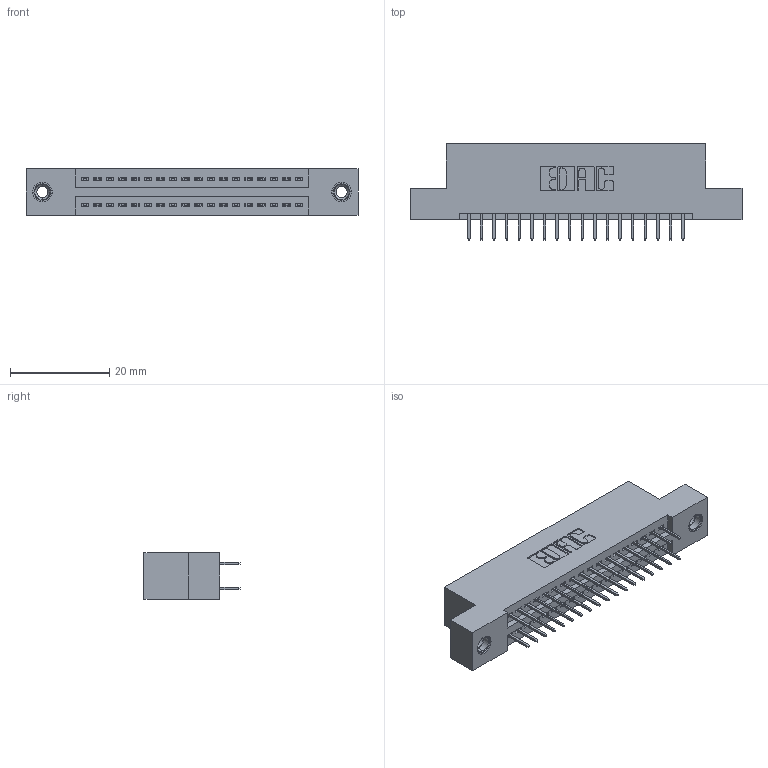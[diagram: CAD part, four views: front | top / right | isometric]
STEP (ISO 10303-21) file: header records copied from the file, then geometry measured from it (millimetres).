
FILE_DESCRIPTION (( 'STEP AP203' ), '1' );
FILE_NAME ('345-036-524-208.STEP', '2018-08-29T10:36:10', ( '' ), ( '' ), 'SwSTEP 2.0', 'SolidWorks 2016', '' );
FILE_SCHEMA (( 'CONFIG_CONTROL_DESIGN' ));
Length unit declared in the file: inch
Products named in the file (4): 345 Part_Flush Mounting Lugs - 0.156 Dia-TI; 345-292-001_345-293-124; 345-250-001_345-250-003-102; 345-036-524-208
Assembly tree (39 placements, depth 2):
  345-036-524-208
    345 Part_Flush Mounting Lugs - 0.156 Dia-TI
    345-292-001_345-293-124  x36
    345-250-001_345-250-003-102  x2
Bounding box: 66.93 x 19.35 x 9.4 mm (x, y, z)
Volume: 6217.8 mm3; surface area: 8595.7 mm2
Topology: 39 solids, 39 shells, 2130 faces, 5985 edges, 3838 vertices
Faces by surface type: plane 1516, cylinder 598, cone 12, torus 4
Entity records: 18614 total; most frequent: CARTESIAN_POINT 3123, ORIENTED_EDGE 3050, DIRECTION 2811, EDGE_CURVE 1525, VECTOR 1305, LINE 1305, VERTEX_POINT 1008, AXIS2_PLACEMENT_3D 753
